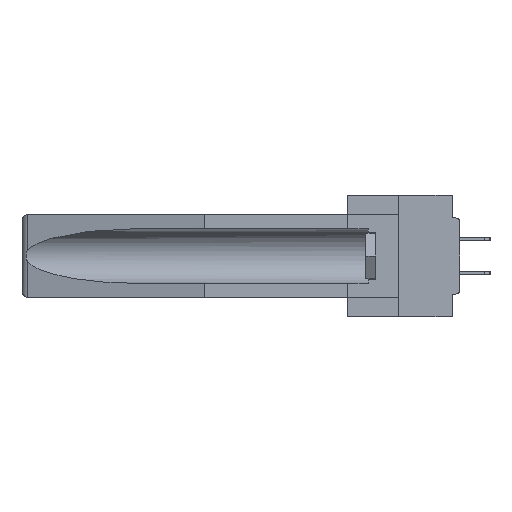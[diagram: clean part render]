
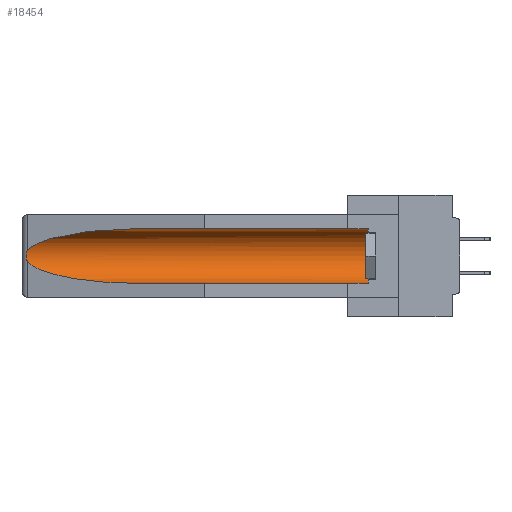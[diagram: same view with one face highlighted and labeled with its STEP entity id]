
A CAD part, left-side view. The second image highlights one B-rep face of the part: STEP entity #18454.
In plain terms, the highlighted cylindrical face has radius 2.857 mm (diameter 5.715 mm), a partial arc.
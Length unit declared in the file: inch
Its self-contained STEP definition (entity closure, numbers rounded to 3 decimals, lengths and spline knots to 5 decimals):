
#177 = CARTESIAN_POINT ( 'NONE',  ( 0.26537, 1.52718, -0.19328 ) ) ;
#393 = ORIENTED_EDGE ( 'NONE', *, *, #29468, .T. ) ;
#513 = VERTEX_POINT ( 'NONE', #18156 ) ;
#1408 = EDGE_CURVE ( 'NONE', #35020, #4486, #10988, .T. ) ;
#2413 = ORIENTED_EDGE ( 'NONE', *, *, #25265, .T. ) ;
#3206 = CARTESIAN_POINT ( 'NONE',  ( 0.21114, 1.30732, -0.284 ) ) ;
#4228 = CARTESIAN_POINT ( 'NONE',  ( 0.155, -0.30754, -0.284 ) ) ;
#4486 = VERTEX_POINT ( 'NONE', #10570 ) ;
#4741 = VERTEX_POINT ( 'NONE', #14483 ) ;
#5463 = CARTESIAN_POINT ( 'NONE',  ( 0.155, 1.07973, -0.059 ) ) ;
#5697 = CARTESIAN_POINT ( 'NONE',  ( 0.26537, 1.52718, -0.19328 ) ) ;
#5780 = CARTESIAN_POINT ( 'NONE',  ( 0.26597, 1.5296, -0.19026 ) ) ;
#5927 = CARTESIAN_POINT ( 'NONE',  ( 0.25451, 1.48313, -0.24835 ) ) ;
#5986 = EDGE_CURVE ( 'NONE', #513, #4486, #28038, .T. ) ;
#6329 = ORIENTED_EDGE ( 'NONE', *, *, #32023, .T. ) ;
#6354 = DIRECTION ( 'NONE',  ( 0., 1., 0. ) ) ;
#6539 = VECTOR ( 'NONE', #6354, 39.37008 ) ;
#8297 = CARTESIAN_POINT ( 'NONE',  ( 0.2675, 1.53308, -0.16763 ) ) ;
#8304 = CARTESIAN_POINT ( 'NONE',  ( 0.155, 0.126, -0.1715 ) ) ;
#8429 = DIRECTION ( 'NONE',  ( 0., -1., 0. ) ) ;
#10570 = CARTESIAN_POINT ( 'NONE',  ( 0.155, 1.07973, -0.284 ) ) ;
#10988 =( BOUNDED_CURVE ( )  B_SPLINE_CURVE ( 3, ( #30219, #5927, #3206, #11060 ),
 .UNSPECIFIED., .F., .F. ) 
 B_SPLINE_CURVE_WITH_KNOTS ( ( 4, 4 ),
 ( 0.1948, 1.5708 ),
 .UNSPECIFIED. ) 
 CURVE ( )  GEOMETRIC_REPRESENTATION_ITEM ( )  RATIONAL_B_SPLINE_CURVE ( ( 1., 0.848, 0.848, 1. ) ) 
 REPRESENTATION_ITEM ( '' )  );
#11026 = CARTESIAN_POINT ( 'NONE',  ( 0.2673, 1.53269, -0.17917 ) ) ;
#11060 = CARTESIAN_POINT ( 'NONE',  ( 0.155, 1.07973, -0.284 ) ) ;
#11620 = FACE_OUTER_BOUND ( 'NONE', #28518, .T. ) ;
#12186 = CARTESIAN_POINT ( 'NONE',  ( 0.155, -0.30754, -0.059 ) ) ;
#13773 = CARTESIAN_POINT ( 'NONE',  ( 0.26537, 1.52718, -0.14972 ) ) ;
#13798 = LINE ( 'NONE', #12186, #6539 ) ;
#14483 = CARTESIAN_POINT ( 'NONE',  ( 0.155, 0.126, -0.059 ) ) ;
#16648 = DIRECTION ( 'NONE',  ( 0., 0., 1. ) ) ;
#16919 = ORIENTED_EDGE ( 'NONE', *, *, #23803, .T. ) ;
#18156 = CARTESIAN_POINT ( 'NONE',  ( 0.155, 0.126, -0.284 ) ) ;
#18454 = ADVANCED_FACE ( 'NONE', ( #11620 ), #21368, .F. ) ;
#19065 = CARTESIAN_POINT ( 'NONE',  ( 0.21114, 1.30732, -0.059 ) ) ;
#20411 = VECTOR ( 'NONE', #34376, 39.37008 ) ;
#20928 = AXIS2_PLACEMENT_3D ( 'NONE', #27632, #27280, #33488 ) ;
#21368 = CYLINDRICAL_SURFACE ( 'NONE', #20928, 0.1125 ) ;
#22146 = B_SPLINE_CURVE_WITH_KNOTS ( 'NONE', 3,
 ( #13773, #24612, #24974, #33192, #8297, #27351, #11026, #32847, #5780, #177 ),
 .UNSPECIFIED., .F., .F.,
 ( 4, 2, 2, 2, 4 ),
 ( 0., 0.00029, 0.00058, 0.00087, 0.00117 ),
 .UNSPECIFIED. ) ;
#22695 = CARTESIAN_POINT ( 'NONE',  ( 0.155, 1.07973, -0.059 ) ) ;
#22853 = AXIS2_PLACEMENT_3D ( 'NONE', #8304, #8429, #16648 ) ;
#23803 = EDGE_CURVE ( 'NONE', #25056, #32838, #34151, .T. ) ;
#24417 = ORIENTED_EDGE ( 'NONE', *, *, #5986, .F. ) ;
#24612 = CARTESIAN_POINT ( 'NONE',  ( 0.26597, 1.52961, -0.15275 ) ) ;
#24974 = CARTESIAN_POINT ( 'NONE',  ( 0.26654, 1.53092, -0.15636 ) ) ;
#25056 = VERTEX_POINT ( 'NONE', #22695 ) ;
#25265 = EDGE_CURVE ( 'NONE', #4741, #25056, #13798, .T. ) ;
#26094 = CARTESIAN_POINT ( 'NONE',  ( 0.26537, 1.52718, -0.14972 ) ) ;
#27280 = DIRECTION ( 'NONE',  ( 0., 1., 0. ) ) ;
#27351 = CARTESIAN_POINT ( 'NONE',  ( 0.2675, 1.53308, -0.17534 ) ) ;
#27632 = CARTESIAN_POINT ( 'NONE',  ( 0.155, -0.30754, -0.1715 ) ) ;
#28038 = LINE ( 'NONE', #4228, #20411 ) ;
#28381 = ORIENTED_EDGE ( 'NONE', *, *, #1408, .T. ) ;
#28518 = EDGE_LOOP ( 'NONE', ( #16919, #393, #28381, #24417, #6329, #2413 ) ) ;
#29468 = EDGE_CURVE ( 'NONE', #32838, #35020, #22146, .T. ) ;
#30219 = CARTESIAN_POINT ( 'NONE',  ( 0.26537, 1.52718, -0.19328 ) ) ;
#30565 = CIRCLE ( 'NONE', #22853, 0.1125 ) ;
#32023 = EDGE_CURVE ( 'NONE', #513, #4741, #30565, .T. ) ;
#32513 = CARTESIAN_POINT ( 'NONE',  ( 0.25451, 1.48313, -0.09465 ) ) ;
#32633 = CARTESIAN_POINT ( 'NONE',  ( 0.26537, 1.52718, -0.14972 ) ) ;
#32838 = VERTEX_POINT ( 'NONE', #26094 ) ;
#32847 = CARTESIAN_POINT ( 'NONE',  ( 0.26655, 1.53094, -0.18657 ) ) ;
#33192 = CARTESIAN_POINT ( 'NONE',  ( 0.2673, 1.5327, -0.16383 ) ) ;
#33488 = DIRECTION ( 'NONE',  ( 0., 0., 1. ) ) ;
#34151 =( BOUNDED_CURVE ( )  B_SPLINE_CURVE ( 3, ( #5463, #19065, #32513, #32633 ),
 .UNSPECIFIED., .F., .T. ) 
 B_SPLINE_CURVE_WITH_KNOTS ( ( 4, 4 ),
 ( 4.71239, 6.08839 ),
 .UNSPECIFIED. ) 
 CURVE ( )  GEOMETRIC_REPRESENTATION_ITEM ( )  RATIONAL_B_SPLINE_CURVE ( ( 1., 0.848, 0.848, 1. ) ) 
 REPRESENTATION_ITEM ( '' )  );
#34376 = DIRECTION ( 'NONE',  ( 0., 1., 0. ) ) ;
#35020 = VERTEX_POINT ( 'NONE', #5697 ) ;
